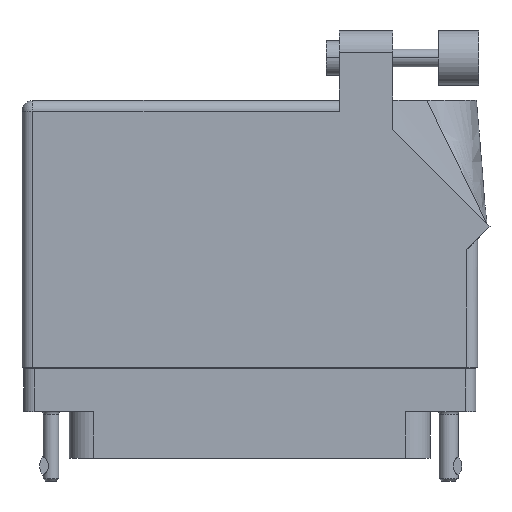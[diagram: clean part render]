
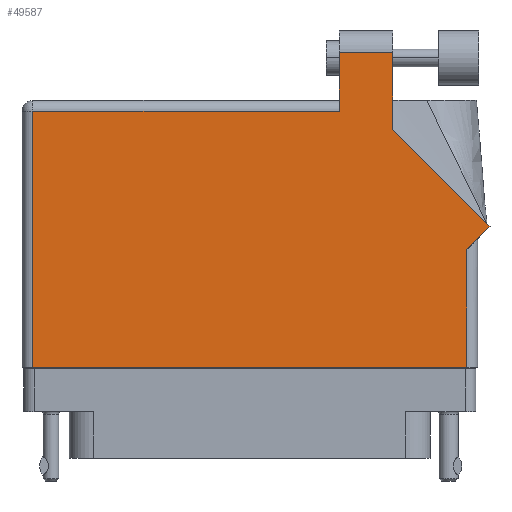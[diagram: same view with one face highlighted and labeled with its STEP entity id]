
A CAD part, front view. The second image highlights one B-rep face of the part: STEP entity #49587.
In plain terms, the highlighted face is planar.
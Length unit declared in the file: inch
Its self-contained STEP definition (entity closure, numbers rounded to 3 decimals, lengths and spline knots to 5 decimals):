
#476 = DIRECTION ( 'NONE',  ( -0.707, 0.707, 0. ) ) ;
#694 = VECTOR ( 'NONE', #43057, 39.37008 ) ;
#731 = CARTESIAN_POINT ( 'NONE',  ( 1.244, -0.1, 0.455 ) ) ;
#910 = VERTEX_POINT ( 'NONE', #61029 ) ;
#2094 = VECTOR ( 'NONE', #35025, 39.37008 ) ;
#2795 = DIRECTION ( 'NONE',  ( 0., -1., 0. ) ) ;
#3505 = VECTOR ( 'NONE', #50437, 39.37008 ) ;
#3582 = PLANE ( 'NONE',  #20810 ) ;
#3799 = LINE ( 'NONE', #10198, #59132 ) ;
#3975 = CARTESIAN_POINT ( 'NONE',  ( -1.306, 1.43, 0.455 ) ) ;
#6168 = EDGE_CURVE ( 'NONE', #41507, #18604, #33660, .T. ) ;
#6785 = ORIENTED_EDGE ( 'NONE', *, *, #9947, .T. ) ;
#7347 = CARTESIAN_POINT ( 'NONE',  ( -1.244, -0.1, 0.455 ) ) ;
#7502 = VERTEX_POINT ( 'NONE', #41949 ) ;
#8524 = CARTESIAN_POINT ( 'NONE',  ( 0.513, 1.705, 0.455 ) ) ;
#9947 = EDGE_CURVE ( 'NONE', #19248, #910, #49356, .T. ) ;
#10198 = CARTESIAN_POINT ( 'NONE',  ( 1.37671, 0.70771, 0.455 ) ) ;
#10621 = VERTEX_POINT ( 'NONE', #53453 ) ;
#10929 = VECTOR ( 'NONE', #31201, 39.37008 ) ;
#12436 = LINE ( 'NONE', #16953, #10929 ) ;
#13066 = ORIENTED_EDGE ( 'NONE', *, *, #25856, .T. ) ;
#13219 = CARTESIAN_POINT ( 'NONE',  ( 0.513, 1.368, 0.455 ) ) ;
#15760 = ORIENTED_EDGE ( 'NONE', *, *, #42051, .T. ) ;
#16605 = VECTOR ( 'NONE', #46028, 39.37008 ) ;
#16953 = CARTESIAN_POINT ( 'NONE',  ( 0.82, 1.26442, 0.455 ) ) ;
#17227 = DIRECTION ( 'NONE',  ( 0., -1., 0. ) ) ;
#18017 = DIRECTION ( 'NONE',  ( 0., 0., -1. ) ) ;
#18604 = VERTEX_POINT ( 'NONE', #50510 ) ;
#19248 = VERTEX_POINT ( 'NONE', #34587 ) ;
#19387 = ORIENTED_EDGE ( 'NONE', *, *, #6168, .T. ) ;
#20810 = AXIS2_PLACEMENT_3D ( 'NONE', #3975, #18017, #36612 ) ;
#21453 = VERTEX_POINT ( 'NONE', #8524 ) ;
#21961 = CARTESIAN_POINT ( 'NONE',  ( -1.306, 1.368, 0.455 ) ) ;
#21996 = CARTESIAN_POINT ( 'NONE',  ( 0.513, 1.43, 0.455 ) ) ;
#22495 = CARTESIAN_POINT ( 'NONE',  ( 0.513, 1.705, 0.455 ) ) ;
#22795 = EDGE_CURVE ( 'NONE', #18604, #25111, #41226, .T. ) ;
#23505 = EDGE_LOOP ( 'NONE', ( #15760, #57549, #46703, #19387, #39504, #24969, #13066, #6785, #40764 ) ) ;
#24969 = ORIENTED_EDGE ( 'NONE', *, *, #43538, .T. ) ;
#25111 = VERTEX_POINT ( 'NONE', #27701 ) ;
#25856 = EDGE_CURVE ( 'NONE', #30796, #19248, #31686, .T. ) ;
#27260 = DIRECTION ( 'NONE',  ( -1., 0., 0. ) ) ;
#27701 = CARTESIAN_POINT ( 'NONE',  ( -1.244, -0.1, 0.455 ) ) ;
#28019 = EDGE_CURVE ( 'NONE', #910, #7502, #3799, .T. ) ;
#28609 = CARTESIAN_POINT ( 'NONE',  ( 1.244, 0.637, 0.455 ) ) ;
#30796 = VERTEX_POINT ( 'NONE', #731 ) ;
#31201 = DIRECTION ( 'NONE',  ( 0., 1., 0. ) ) ;
#31225 = VECTOR ( 'NONE', #17227, 39.37008 ) ;
#31686 = LINE ( 'NONE', #28609, #694 ) ;
#33660 = LINE ( 'NONE', #21961, #3505 ) ;
#34587 = CARTESIAN_POINT ( 'NONE',  ( 1.244, 0.575, 0.455 ) ) ;
#35025 = DIRECTION ( 'NONE',  ( 0.707, 0.707, 0. ) ) ;
#36612 = DIRECTION ( 'NONE',  ( -1., 0., 0. ) ) ;
#39504 = ORIENTED_EDGE ( 'NONE', *, *, #22795, .T. ) ;
#40764 = ORIENTED_EDGE ( 'NONE', *, *, #28019, .T. ) ;
#41077 = CARTESIAN_POINT ( 'NONE',  ( -1.306, -0.1, 0.455 ) ) ;
#41226 = LINE ( 'NONE', #7347, #42654 ) ;
#41507 = VERTEX_POINT ( 'NONE', #13219 ) ;
#41949 = CARTESIAN_POINT ( 'NONE',  ( 0.82, 1.26442, 0.455 ) ) ;
#42051 = EDGE_CURVE ( 'NONE', #7502, #10621, #12436, .T. ) ;
#42654 = VECTOR ( 'NONE', #2795, 39.37008 ) ;
#43057 = DIRECTION ( 'NONE',  ( 0., 1., 0. ) ) ;
#43538 = EDGE_CURVE ( 'NONE', #25111, #30796, #46872, .T. ) ;
#46028 = DIRECTION ( 'NONE',  ( 1., 0., 0. ) ) ;
#46703 = ORIENTED_EDGE ( 'NONE', *, *, #48903, .T. ) ;
#46872 = LINE ( 'NONE', #41077, #16605 ) ;
#48903 = EDGE_CURVE ( 'NONE', #21453, #41507, #53333, .T. ) ;
#49356 = LINE ( 'NONE', #54375, #2094 ) ;
#49587 = ADVANCED_FACE ( 'NONE', ( #60581 ), #3582, .F. ) ;
#50437 = DIRECTION ( 'NONE',  ( -1., 0., 0. ) ) ;
#50510 = CARTESIAN_POINT ( 'NONE',  ( -1.244, 1.368, 0.455 ) ) ;
#53333 = LINE ( 'NONE', #21996, #31225 ) ;
#53453 = CARTESIAN_POINT ( 'NONE',  ( 0.82, 1.705, 0.455 ) ) ;
#54375 = CARTESIAN_POINT ( 'NONE',  ( 1.306, 0.637, 0.455 ) ) ;
#54786 = LINE ( 'NONE', #22495, #56284 ) ;
#56284 = VECTOR ( 'NONE', #27260, 39.37008 ) ;
#57549 = ORIENTED_EDGE ( 'NONE', *, *, #58541, .T. ) ;
#58541 = EDGE_CURVE ( 'NONE', #10621, #21453, #54786, .T. ) ;
#59132 = VECTOR ( 'NONE', #476, 39.37008 ) ;
#60581 = FACE_OUTER_BOUND ( 'NONE', #23505, .T. ) ;
#61029 = CARTESIAN_POINT ( 'NONE',  ( 1.37671, 0.70771, 0.455 ) ) ;
